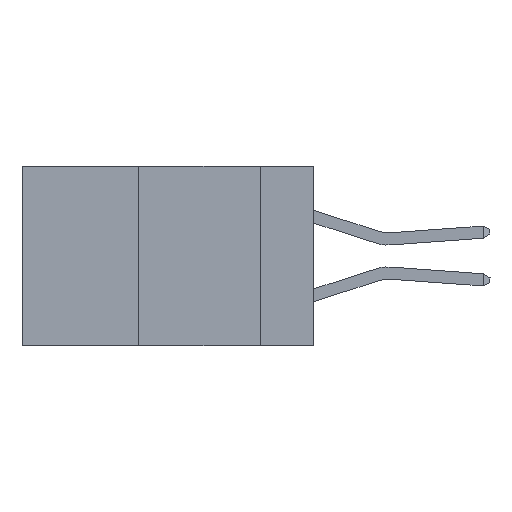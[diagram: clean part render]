
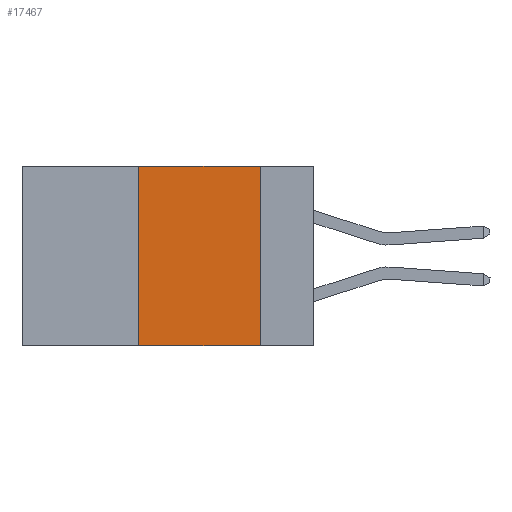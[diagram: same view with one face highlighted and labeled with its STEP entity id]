
A CAD part, left-side view. The second image highlights one B-rep face of the part: STEP entity #17467.
In plain terms, the highlighted planar face has unit normal (-1, 0, 0).
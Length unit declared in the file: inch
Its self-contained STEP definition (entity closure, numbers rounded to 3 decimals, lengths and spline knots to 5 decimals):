
#499 = CARTESIAN_POINT ( 'NONE',  ( 0., 0.6, 0. ) ) ;
#882 = CARTESIAN_POINT ( 'NONE',  ( 0., 0.11, -0.37 ) ) ;
#2056 = FACE_OUTER_BOUND ( 'NONE', #14921, .T. ) ;
#2896 = VECTOR ( 'NONE', #4408, 39.37008 ) ;
#3692 = DIRECTION ( 'NONE',  ( 1., 0., 0. ) ) ;
#4408 = DIRECTION ( 'NONE',  ( 0., -1., 0. ) ) ;
#5849 = VERTEX_POINT ( 'NONE', #16198 ) ;
#7963 = VECTOR ( 'NONE', #11517, 39.37008 ) ;
#10006 = VERTEX_POINT ( 'NONE', #42745 ) ;
#11183 = LINE ( 'NONE', #499, #2896 ) ;
#11517 = DIRECTION ( 'NONE',  ( 0., 0., -1. ) ) ;
#12292 = ORIENTED_EDGE ( 'NONE', *, *, #34070, .F. ) ;
#13124 = LINE ( 'NONE', #20739, #13667 ) ;
#13667 = VECTOR ( 'NONE', #17542, 39.37008 ) ;
#14565 = CARTESIAN_POINT ( 'NONE',  ( 0., 0.11, 0. ) ) ;
#14921 = EDGE_LOOP ( 'NONE', ( #12292, #25487, #40289, #18357 ) ) ;
#16198 = CARTESIAN_POINT ( 'NONE',  ( 0., 0.11, 0. ) ) ;
#16328 = VERTEX_POINT ( 'NONE', #882 ) ;
#17467 = ADVANCED_FACE ( 'NONE', ( #2056 ), #23669, .F. ) ;
#17474 = LINE ( 'NONE', #21283, #25252 ) ;
#17542 = DIRECTION ( 'NONE',  ( 0., 0., 1. ) ) ;
#17970 = DIRECTION ( 'NONE',  ( 0., -1., 0. ) ) ;
#18357 = ORIENTED_EDGE ( 'NONE', *, *, #19081, .T. ) ;
#18360 = CARTESIAN_POINT ( 'NONE',  ( 0., 0.36, -0.37 ) ) ;
#19001 = AXIS2_PLACEMENT_3D ( 'NONE', #23526, #3692, #30188 ) ;
#19081 = EDGE_CURVE ( 'NONE', #29263, #16328, #17474, .T. ) ;
#20739 = CARTESIAN_POINT ( 'NONE',  ( 0., 0.36, 0. ) ) ;
#21283 = CARTESIAN_POINT ( 'NONE',  ( 0., 0.6, -0.37 ) ) ;
#23526 = CARTESIAN_POINT ( 'NONE',  ( 0., 0.6, 0. ) ) ;
#23669 = PLANE ( 'NONE',  #19001 ) ;
#24471 = EDGE_CURVE ( 'NONE', #10006, #5849, #11183, .T. ) ;
#25252 = VECTOR ( 'NONE', #17970, 39.37008 ) ;
#25487 = ORIENTED_EDGE ( 'NONE', *, *, #24471, .F. ) ;
#26618 = LINE ( 'NONE', #14565, #7963 ) ;
#29263 = VERTEX_POINT ( 'NONE', #18360 ) ;
#30188 = DIRECTION ( 'NONE',  ( 0., 0., -1. ) ) ;
#34070 = EDGE_CURVE ( 'NONE', #5849, #16328, #26618, .T. ) ;
#40289 = ORIENTED_EDGE ( 'NONE', *, *, #41260, .F. ) ;
#41260 = EDGE_CURVE ( 'NONE', #29263, #10006, #13124, .T. ) ;
#42745 = CARTESIAN_POINT ( 'NONE',  ( 0., 0.36, 0. ) ) ;
